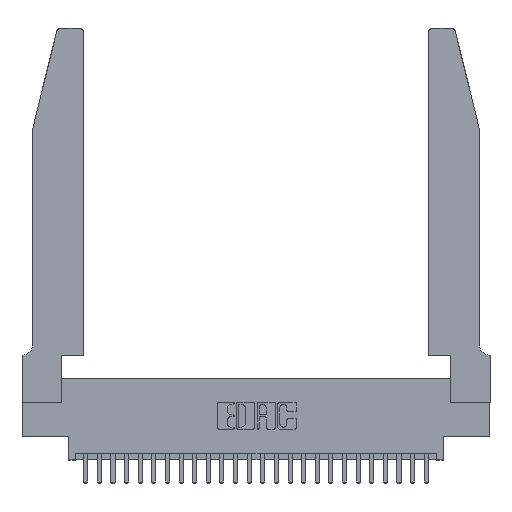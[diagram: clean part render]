
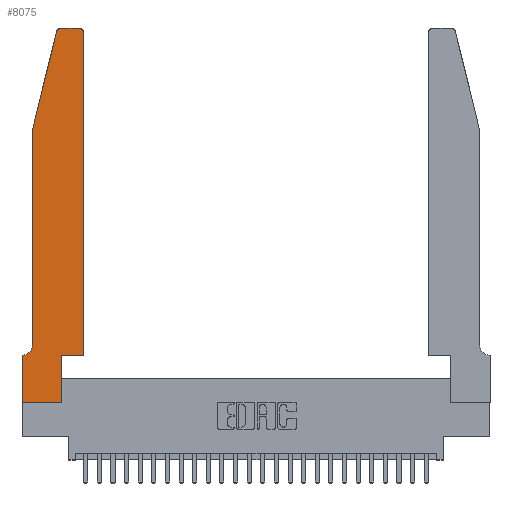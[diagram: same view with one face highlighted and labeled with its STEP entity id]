
A CAD part, top view. The second image highlights one B-rep face of the part: STEP entity #8075.
In plain terms, the highlighted planar face has unit normal (0, 0, 1).
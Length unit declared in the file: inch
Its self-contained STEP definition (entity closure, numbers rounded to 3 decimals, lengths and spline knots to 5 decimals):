
#71 = DIRECTION ( 'NONE',  ( -0.239, -0.971, 0. ) ) ;
#269 = PLANE ( 'NONE',  #7012 ) ;
#1536 = DIRECTION ( 'NONE',  ( 1., 0., 0. ) ) ;
#1923 = FACE_OUTER_BOUND ( 'NONE', #5568, .T. ) ;
#2057 = DIRECTION ( 'NONE',  ( 0., -1., 0. ) ) ;
#2132 = VECTOR ( 'NONE', #15605, 39.37008 ) ;
#2346 = VECTOR ( 'NONE', #19836, 39.37008 ) ;
#2419 = CARTESIAN_POINT ( 'NONE',  ( 0.284, 2.75, 0.37 ) ) ;
#2492 = CARTESIAN_POINT ( 'NONE',  ( 0.0755, 2., 0.37 ) ) ;
#2635 = ORIENTED_EDGE ( 'NONE', *, *, #21834, .T. ) ;
#2707 = CARTESIAN_POINT ( 'NONE',  ( 0.0755, 0.35, 0.37 ) ) ;
#3100 = DIRECTION ( 'NONE',  ( -1., 0., 0. ) ) ;
#3128 = EDGE_CURVE ( 'NONE', #9114, #9099, #4990, .T. ) ;
#3737 = VERTEX_POINT ( 'NONE', #8653 ) ;
#3774 = CARTESIAN_POINT ( 'NONE',  ( 0.0755, 2., 0.37 ) ) ;
#3844 = AXIS2_PLACEMENT_3D ( 'NONE', #9809, #24718, #7943 ) ;
#4342 = ORIENTED_EDGE ( 'NONE', *, *, #15520, .T. ) ;
#4541 = ORIENTED_EDGE ( 'NONE', *, *, #19642, .T. ) ;
#4577 = CARTESIAN_POINT ( 'NONE',  ( 0.0755, 2., 0.37 ) ) ;
#4974 = CARTESIAN_POINT ( 'NONE',  ( 0.2865, 0.35, 0.37 ) ) ;
#4990 = LINE ( 'NONE', #23036, #22651 ) ;
#5036 = ORIENTED_EDGE ( 'NONE', *, *, #5888, .T. ) ;
#5513 = LINE ( 'NONE', #2707, #20470 ) ;
#5568 = EDGE_LOOP ( 'NONE', ( #18771, #23853, #17769, #2635, #5036, #4541, #18613, #24914, #10562, #26849, #11501, #4342 ) ) ;
#5888 = EDGE_CURVE ( 'NONE', #16791, #8016, #7692, .T. ) ;
#6570 = DIRECTION ( 'NONE',  ( 0., -1., 0. ) ) ;
#6911 = DIRECTION ( 'NONE',  ( 1., 0., 0. ) ) ;
#6983 = CARTESIAN_POINT ( 'NONE',  ( 0.4505, 0.35, 0.37 ) ) ;
#7003 = DIRECTION ( 'NONE',  ( -1., 0., 0. ) ) ;
#7012 = AXIS2_PLACEMENT_3D ( 'NONE', #10914, #21697, #6911 ) ;
#7632 = LINE ( 'NONE', #4974, #2346 ) ;
#7692 = CIRCLE ( 'NONE', #9830, 0.07 ) ;
#7845 = CARTESIAN_POINT ( 'NONE',  ( 0., 0., 0.37 ) ) ;
#7943 = DIRECTION ( 'NONE',  ( 1., 0., 0. ) ) ;
#8016 = VERTEX_POINT ( 'NONE', #8934 ) ;
#8075 = ADVANCED_FACE ( 'NONE', ( #1923 ), #269, .T. ) ;
#8242 = CARTESIAN_POINT ( 'NONE',  ( 0.4205, 2.72, 0.37 ) ) ;
#8550 = EDGE_CURVE ( 'NONE', #3737, #26272, #26533, .T. ) ;
#8653 = CARTESIAN_POINT ( 'NONE',  ( 0.25487, 2.72718, 0.37 ) ) ;
#8934 = CARTESIAN_POINT ( 'NONE',  ( 0.0055, 0.35, 0.37 ) ) ;
#9099 = VERTEX_POINT ( 'NONE', #17745 ) ;
#9114 = VERTEX_POINT ( 'NONE', #15338 ) ;
#9401 = CARTESIAN_POINT ( 'NONE',  ( 0.0055, 0.42, 0.37 ) ) ;
#9809 = CARTESIAN_POINT ( 'NONE',  ( 0.284, 2.72, 0.37 ) ) ;
#9830 = AXIS2_PLACEMENT_3D ( 'NONE', #9401, #20210, #3100 ) ;
#10403 = DIRECTION ( 'NONE',  ( 0., 0., 1. ) ) ;
#10558 = CIRCLE ( 'NONE', #25174, 0.03 ) ;
#10562 = ORIENTED_EDGE ( 'NONE', *, *, #14059, .T. ) ;
#10778 = EDGE_CURVE ( 'NONE', #14976, #3737, #25456, .T. ) ;
#10914 = CARTESIAN_POINT ( 'NONE',  ( 0., 0.35, 0.37 ) ) ;
#11033 = VERTEX_POINT ( 'NONE', #22661 ) ;
#11467 = VERTEX_POINT ( 'NONE', #11627 ) ;
#11501 = ORIENTED_EDGE ( 'NONE', *, *, #3128, .T. ) ;
#11627 = CARTESIAN_POINT ( 'NONE',  ( 0., 0., 0.37 ) ) ;
#12096 = EDGE_CURVE ( 'NONE', #20609, #9114, #13401, .T. ) ;
#12936 = CARTESIAN_POINT ( 'NONE',  ( 0.4205, 2.75, 0.37 ) ) ;
#13037 = DIRECTION ( 'NONE',  ( 0., 1., 0. ) ) ;
#13401 = LINE ( 'NONE', #6983, #2132 ) ;
#14059 = EDGE_CURVE ( 'NONE', #16471, #20609, #7632, .T. ) ;
#14415 = VERTEX_POINT ( 'NONE', #12936 ) ;
#14689 = VECTOR ( 'NONE', #6570, 39.37008 ) ;
#14976 = VERTEX_POINT ( 'NONE', #2419 ) ;
#15282 = VECTOR ( 'NONE', #2057, 39.37008 ) ;
#15338 = CARTESIAN_POINT ( 'NONE',  ( 0.4505, 0.35, 0.37 ) ) ;
#15520 = EDGE_CURVE ( 'NONE', #9099, #14415, #10558, .T. ) ;
#15605 = DIRECTION ( 'NONE',  ( 1., 0., 0. ) ) ;
#15679 = DIRECTION ( 'NONE',  ( -1., 0., 0. ) ) ;
#15801 = CARTESIAN_POINT ( 'NONE',  ( 0.2865, 0., 0.37 ) ) ;
#16471 = VERTEX_POINT ( 'NONE', #15801 ) ;
#16791 = VERTEX_POINT ( 'NONE', #21772 ) ;
#17178 = VECTOR ( 'NONE', #7003, 39.37008 ) ;
#17745 = CARTESIAN_POINT ( 'NONE',  ( 0.4505, 2.72, 0.37 ) ) ;
#17769 = ORIENTED_EDGE ( 'NONE', *, *, #8550, .T. ) ;
#18243 = VECTOR ( 'NONE', #1536, 39.37008 ) ;
#18549 = LINE ( 'NONE', #19996, #17178 ) ;
#18613 = ORIENTED_EDGE ( 'NONE', *, *, #22988, .T. ) ;
#18771 = ORIENTED_EDGE ( 'NONE', *, *, #26755, .T. ) ;
#19642 = EDGE_CURVE ( 'NONE', #8016, #11033, #5513, .T. ) ;
#19836 = DIRECTION ( 'NONE',  ( 0., 1., 0. ) ) ;
#19996 = CARTESIAN_POINT ( 'NONE',  ( 0.2605, 2.75, 0.37 ) ) ;
#20210 = DIRECTION ( 'NONE',  ( 0., 0., -1. ) ) ;
#20470 = VECTOR ( 'NONE', #15679, 39.37008 ) ;
#20609 = VERTEX_POINT ( 'NONE', #23745 ) ;
#21697 = DIRECTION ( 'NONE',  ( 0., 0., 1. ) ) ;
#21772 = CARTESIAN_POINT ( 'NONE',  ( 0.0755, 0.42, 0.37 ) ) ;
#21834 = EDGE_CURVE ( 'NONE', #26272, #16791, #25706, .T. ) ;
#22651 = VECTOR ( 'NONE', #13037, 39.37008 ) ;
#22661 = CARTESIAN_POINT ( 'NONE',  ( 0., 0.35, 0.37 ) ) ;
#22944 = LINE ( 'NONE', #7845, #18243 ) ;
#22988 = EDGE_CURVE ( 'NONE', #11033, #11467, #25981, .T. ) ;
#23036 = CARTESIAN_POINT ( 'NONE',  ( 0.4505, 0.35, 0.37 ) ) ;
#23260 = CARTESIAN_POINT ( 'NONE',  ( 0., 0., 0.37 ) ) ;
#23745 = CARTESIAN_POINT ( 'NONE',  ( 0.2865, 0.35, 0.37 ) ) ;
#23853 = ORIENTED_EDGE ( 'NONE', *, *, #10778, .T. ) ;
#23874 = VECTOR ( 'NONE', #71, 39.37008 ) ;
#24071 = EDGE_CURVE ( 'NONE', #11467, #16471, #22944, .T. ) ;
#24718 = DIRECTION ( 'NONE',  ( 0., 0., 1. ) ) ;
#24914 = ORIENTED_EDGE ( 'NONE', *, *, #24071, .T. ) ;
#25174 = AXIS2_PLACEMENT_3D ( 'NONE', #8242, #10403, #25314 ) ;
#25314 = DIRECTION ( 'NONE',  ( 1., 0., 0. ) ) ;
#25456 = CIRCLE ( 'NONE', #3844, 0.03 ) ;
#25706 = LINE ( 'NONE', #2492, #14689 ) ;
#25981 = LINE ( 'NONE', #23260, #15282 ) ;
#26272 = VERTEX_POINT ( 'NONE', #3774 ) ;
#26533 = LINE ( 'NONE', #4577, #23874 ) ;
#26755 = EDGE_CURVE ( 'NONE', #14415, #14976, #18549, .T. ) ;
#26849 = ORIENTED_EDGE ( 'NONE', *, *, #12096, .T. ) ;
